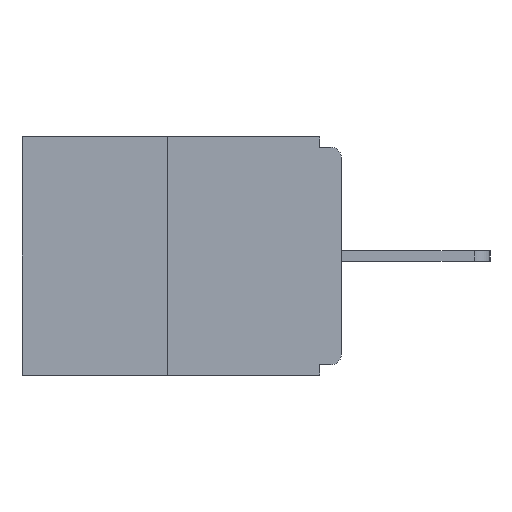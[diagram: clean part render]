
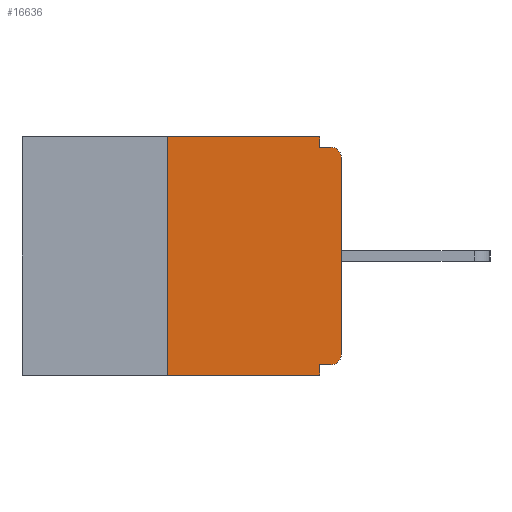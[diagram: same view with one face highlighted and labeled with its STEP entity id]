
A CAD part, left-side view. The second image highlights one B-rep face of the part: STEP entity #16636.
In plain terms, the highlighted planar face has unit normal (-1, 0, 0).
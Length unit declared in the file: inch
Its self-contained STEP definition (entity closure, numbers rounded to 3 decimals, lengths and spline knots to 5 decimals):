
#169 = VERTEX_POINT ( 'NONE', #13150 ) ;
#240 = EDGE_CURVE ( 'NONE', #169, #8257, #6062, .T. ) ;
#679 = CARTESIAN_POINT ( 'NONE',  ( 0., 0.46, 0. ) ) ;
#737 = VECTOR ( 'NONE', #14586, 39.37008 ) ;
#982 = DIRECTION ( 'NONE',  ( 1., 0., 0. ) ) ;
#1014 = ORIENTED_EDGE ( 'NONE', *, *, #19234, .F. ) ;
#1070 = EDGE_LOOP ( 'NONE', ( #6536, #5197, #10526, #18212, #9757, #18202, #16406, #17910, #1014, #9075 ) ) ;
#1203 = LINE ( 'NONE', #12279, #3437 ) ;
#1405 = VERTEX_POINT ( 'NONE', #16565 ) ;
#1781 = EDGE_CURVE ( 'NONE', #18970, #14397, #3819, .T. ) ;
#1810 = CARTESIAN_POINT ( 'NONE',  ( 0., 0.46, -0.343 ) ) ;
#1814 = EDGE_CURVE ( 'NONE', #19785, #169, #7851, .T. ) ;
#1823 = CARTESIAN_POINT ( 'NONE',  ( 0., 0., -0.328 ) ) ;
#2383 = VERTEX_POINT ( 'NONE', #18667 ) ;
#3437 = VECTOR ( 'NONE', #10633, 39.37008 ) ;
#3819 = LINE ( 'NONE', #11406, #737 ) ;
#4018 = CARTESIAN_POINT ( 'NONE',  ( 0., 0.015, -0.313 ) ) ;
#4202 = VERTEX_POINT ( 'NONE', #9797 ) ;
#5140 = DIRECTION ( 'NONE',  ( -1., 0., 0. ) ) ;
#5197 = ORIENTED_EDGE ( 'NONE', *, *, #11681, .F. ) ;
#5399 = VECTOR ( 'NONE', #17640, 39.37008 ) ;
#5911 = VERTEX_POINT ( 'NONE', #13160 ) ;
#6062 = LINE ( 'NONE', #8926, #17973 ) ;
#6065 = LINE ( 'NONE', #18697, #14073 ) ;
#6153 = CIRCLE ( 'NONE', #17641, 0.015 ) ;
#6536 = ORIENTED_EDGE ( 'NONE', *, *, #9314, .F. ) ;
#7260 = CARTESIAN_POINT ( 'NONE',  ( 0., 0.031, -0.015 ) ) ;
#7386 = DIRECTION ( 'NONE',  ( 0., -1., 0. ) ) ;
#7497 = CARTESIAN_POINT ( 'NONE',  ( 0., 0.015, -0.03 ) ) ;
#7851 = CIRCLE ( 'NONE', #9203, 0.015 ) ;
#8257 = VERTEX_POINT ( 'NONE', #9427 ) ;
#8766 = PLANE ( 'NONE',  #18166 ) ;
#8871 = CARTESIAN_POINT ( 'NONE',  ( 0., 0.031, 0. ) ) ;
#8926 = CARTESIAN_POINT ( 'NONE',  ( 0., 0., 0. ) ) ;
#9033 = DIRECTION ( 'NONE',  ( -1., 0., 0. ) ) ;
#9034 = DIRECTION ( 'NONE',  ( 0., 0., 1. ) ) ;
#9075 = ORIENTED_EDGE ( 'NONE', *, *, #1781, .F. ) ;
#9203 = AXIS2_PLACEMENT_3D ( 'NONE', #4018, #5140, #19506 ) ;
#9314 = EDGE_CURVE ( 'NONE', #1405, #18970, #15311, .T. ) ;
#9427 = CARTESIAN_POINT ( 'NONE',  ( 0., 0., -0.03 ) ) ;
#9727 = VECTOR ( 'NONE', #7386, 39.37008 ) ;
#9757 = ORIENTED_EDGE ( 'NONE', *, *, #16015, .F. ) ;
#9797 = CARTESIAN_POINT ( 'NONE',  ( 0., 0.031, -0.328 ) ) ;
#10372 = CARTESIAN_POINT ( 'NONE',  ( 0., 0.46, 0. ) ) ;
#10412 = EDGE_CURVE ( 'NONE', #8257, #5911, #6153, .T. ) ;
#10526 = ORIENTED_EDGE ( 'NONE', *, *, #18928, .T. ) ;
#10615 = LINE ( 'NONE', #17202, #11687 ) ;
#10633 = DIRECTION ( 'NONE',  ( 0., 0., -1. ) ) ;
#10859 = VERTEX_POINT ( 'NONE', #18669 ) ;
#11406 = CARTESIAN_POINT ( 'NONE',  ( 0., 0.031, 0. ) ) ;
#11681 = EDGE_CURVE ( 'NONE', #2383, #1405, #6065, .T. ) ;
#11687 = VECTOR ( 'NONE', #15663, 39.37008 ) ;
#12279 = CARTESIAN_POINT ( 'NONE',  ( 0., 0.031, -0.343 ) ) ;
#12888 = DIRECTION ( 'NONE',  ( 0., -1., 0. ) ) ;
#13150 = CARTESIAN_POINT ( 'NONE',  ( 0., 0., -0.313 ) ) ;
#13160 = CARTESIAN_POINT ( 'NONE',  ( 0., 0.015, -0.015 ) ) ;
#14073 = VECTOR ( 'NONE', #17074, 39.37008 ) ;
#14240 = LINE ( 'NONE', #1810, #19540 ) ;
#14397 = VERTEX_POINT ( 'NONE', #7260 ) ;
#14586 = DIRECTION ( 'NONE',  ( 0., 0., -1. ) ) ;
#14638 = FACE_OUTER_BOUND ( 'NONE', #1070, .T. ) ;
#15311 = LINE ( 'NONE', #10372, #9727 ) ;
#15622 = DIRECTION ( 'NONE',  ( 0., 0., -1. ) ) ;
#15663 = DIRECTION ( 'NONE',  ( 0., -1., 0. ) ) ;
#16015 = EDGE_CURVE ( 'NONE', #19785, #4202, #19170, .T. ) ;
#16389 = DIRECTION ( 'NONE',  ( 0., 0., -1. ) ) ;
#16406 = ORIENTED_EDGE ( 'NONE', *, *, #240, .T. ) ;
#16565 = CARTESIAN_POINT ( 'NONE',  ( 0., 0.25, 0. ) ) ;
#16636 = ADVANCED_FACE ( 'NONE', ( #14638 ), #8766, .F. ) ;
#17074 = DIRECTION ( 'NONE',  ( 0., 0., 1. ) ) ;
#17202 = CARTESIAN_POINT ( 'NONE',  ( 0., 0., -0.015 ) ) ;
#17553 = EDGE_CURVE ( 'NONE', #4202, #10859, #1203, .T. ) ;
#17640 = DIRECTION ( 'NONE',  ( 0., 1., 0. ) ) ;
#17641 = AXIS2_PLACEMENT_3D ( 'NONE', #7497, #9033, #15622 ) ;
#17910 = ORIENTED_EDGE ( 'NONE', *, *, #10412, .T. ) ;
#17973 = VECTOR ( 'NONE', #9034, 39.37008 ) ;
#18166 = AXIS2_PLACEMENT_3D ( 'NONE', #679, #982, #16389 ) ;
#18202 = ORIENTED_EDGE ( 'NONE', *, *, #1814, .T. ) ;
#18212 = ORIENTED_EDGE ( 'NONE', *, *, #17553, .F. ) ;
#18667 = CARTESIAN_POINT ( 'NONE',  ( 0., 0.25, -0.343 ) ) ;
#18669 = CARTESIAN_POINT ( 'NONE',  ( 0., 0.031, -0.343 ) ) ;
#18697 = CARTESIAN_POINT ( 'NONE',  ( 0., 0.25, 0. ) ) ;
#18928 = EDGE_CURVE ( 'NONE', #2383, #10859, #14240, .T. ) ;
#18970 = VERTEX_POINT ( 'NONE', #8871 ) ;
#19170 = LINE ( 'NONE', #1823, #5399 ) ;
#19216 = CARTESIAN_POINT ( 'NONE',  ( 0., 0.015, -0.328 ) ) ;
#19234 = EDGE_CURVE ( 'NONE', #14397, #5911, #10615, .T. ) ;
#19506 = DIRECTION ( 'NONE',  ( 0., 0., -1. ) ) ;
#19540 = VECTOR ( 'NONE', #12888, 39.37008 ) ;
#19785 = VERTEX_POINT ( 'NONE', #19216 ) ;
